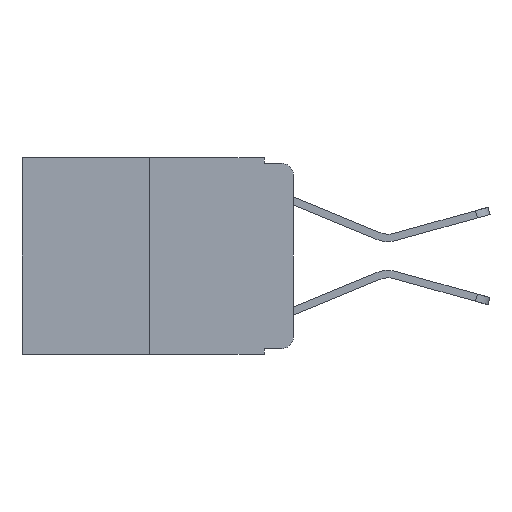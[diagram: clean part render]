
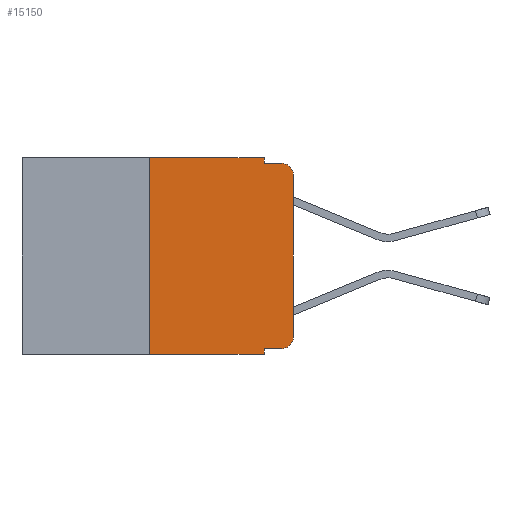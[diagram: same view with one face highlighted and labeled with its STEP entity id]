
A CAD part, left-side view. The second image highlights one B-rep face of the part: STEP entity #15150.
In plain terms, the highlighted planar face has unit normal (-1, 0, 0).
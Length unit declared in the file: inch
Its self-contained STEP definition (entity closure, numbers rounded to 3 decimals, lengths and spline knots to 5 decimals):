
#358 = FACE_OUTER_BOUND ( 'NONE', #2699, .T. ) ;
#746 = CARTESIAN_POINT ( 'NONE',  ( 0., 0., -0.03 ) ) ;
#933 = VECTOR ( 'NONE', #9286, 39.37008 ) ;
#1063 = VERTEX_POINT ( 'NONE', #14488 ) ;
#1134 = CARTESIAN_POINT ( 'NONE',  ( 0., 0.051, -0.01 ) ) ;
#1545 = VERTEX_POINT ( 'NONE', #13090 ) ;
#1669 = ORIENTED_EDGE ( 'NONE', *, *, #3342, .F. ) ;
#2285 = DIRECTION ( 'NONE',  ( 0., -1., 0. ) ) ;
#2361 = CARTESIAN_POINT ( 'NONE',  ( 0., 0.051, -0.343 ) ) ;
#2459 = VERTEX_POINT ( 'NONE', #11951 ) ;
#2699 = EDGE_LOOP ( 'NONE', ( #15648, #10214, #8199, #13859, #8442, #6849, #11143, #1669, #5261, #14802 ) ) ;
#2815 = CARTESIAN_POINT ( 'NONE',  ( 0., 0.25, 0. ) ) ;
#2827 = VECTOR ( 'NONE', #3890, 39.37008 ) ;
#3004 = VECTOR ( 'NONE', #3378, 39.37008 ) ;
#3108 = CARTESIAN_POINT ( 'NONE',  ( 0., 0.473, 0. ) ) ;
#3288 = LINE ( 'NONE', #3391, #2827 ) ;
#3289 = LINE ( 'NONE', #15414, #18353 ) ;
#3342 = EDGE_CURVE ( 'NONE', #17640, #17382, #3288, .T. ) ;
#3378 = DIRECTION ( 'NONE',  ( 0., -1., 0. ) ) ;
#3391 = CARTESIAN_POINT ( 'NONE',  ( 0., 0.051, 0. ) ) ;
#3419 = CARTESIAN_POINT ( 'NONE',  ( 0., 0.051, -0.333 ) ) ;
#3674 = VECTOR ( 'NONE', #11864, 39.37008 ) ;
#3890 = DIRECTION ( 'NONE',  ( 0., 0., -1. ) ) ;
#3921 = VERTEX_POINT ( 'NONE', #12696 ) ;
#4242 = EDGE_CURVE ( 'NONE', #14342, #2459, #15188, .T. ) ;
#4639 = DIRECTION ( 'NONE',  ( 0., 0., -1. ) ) ;
#4884 = AXIS2_PLACEMENT_3D ( 'NONE', #5359, #15498, #6832 ) ;
#4999 = CIRCLE ( 'NONE', #16912, 0.02 ) ;
#5261 = ORIENTED_EDGE ( 'NONE', *, *, #16424, .T. ) ;
#5298 = LINE ( 'NONE', #17523, #16865 ) ;
#5359 = CARTESIAN_POINT ( 'NONE',  ( 0., 0.02, -0.313 ) ) ;
#5643 = EDGE_CURVE ( 'NONE', #11646, #17382, #14668, .T. ) ;
#6179 = VECTOR ( 'NONE', #17844, 39.37008 ) ;
#6579 = CARTESIAN_POINT ( 'NONE',  ( 0., 0.02, -0.03 ) ) ;
#6627 = LINE ( 'NONE', #7706, #6179 ) ;
#6832 = DIRECTION ( 'NONE',  ( 0., 0., -1. ) ) ;
#6849 = ORIENTED_EDGE ( 'NONE', *, *, #7326, .F. ) ;
#7065 = CIRCLE ( 'NONE', #4884, 0.02 ) ;
#7326 = EDGE_CURVE ( 'NONE', #11646, #14342, #5298, .T. ) ;
#7594 = CARTESIAN_POINT ( 'NONE',  ( 0., 0.473, 0. ) ) ;
#7706 = CARTESIAN_POINT ( 'NONE',  ( 0., 0., 0. ) ) ;
#8043 = DIRECTION ( 'NONE',  ( 0., 0., -1. ) ) ;
#8199 = ORIENTED_EDGE ( 'NONE', *, *, #14121, .F. ) ;
#8440 = LINE ( 'NONE', #3419, #933 ) ;
#8442 = ORIENTED_EDGE ( 'NONE', *, *, #4242, .F. ) ;
#8975 = CARTESIAN_POINT ( 'NONE',  ( 0., 0.473, -0.343 ) ) ;
#9242 = EDGE_CURVE ( 'NONE', #3921, #15305, #6627, .T. ) ;
#9286 = DIRECTION ( 'NONE',  ( 0., -1., 0. ) ) ;
#9549 = CARTESIAN_POINT ( 'NONE',  ( 0., 0.25, -0.343 ) ) ;
#10214 = ORIENTED_EDGE ( 'NONE', *, *, #13421, .T. ) ;
#10243 = EDGE_CURVE ( 'NONE', #2459, #17505, #11917, .T. ) ;
#10300 = DIRECTION ( 'NONE',  ( 0., 0., 1. ) ) ;
#11143 = ORIENTED_EDGE ( 'NONE', *, *, #5643, .T. ) ;
#11335 = VECTOR ( 'NONE', #16847, 39.37008 ) ;
#11646 = VERTEX_POINT ( 'NONE', #9549 ) ;
#11864 = DIRECTION ( 'NONE',  ( 0., 0., -1. ) ) ;
#11894 = PLANE ( 'NONE',  #12833 ) ;
#11917 = LINE ( 'NONE', #14787, #3674 ) ;
#11951 = CARTESIAN_POINT ( 'NONE',  ( 0., 0.051, 0. ) ) ;
#12696 = CARTESIAN_POINT ( 'NONE',  ( 0., 0., -0.313 ) ) ;
#12833 = AXIS2_PLACEMENT_3D ( 'NONE', #3108, #13369, #4639 ) ;
#13090 = CARTESIAN_POINT ( 'NONE',  ( 0., 0.02, -0.333 ) ) ;
#13369 = DIRECTION ( 'NONE',  ( 1., 0., 0. ) ) ;
#13421 = EDGE_CURVE ( 'NONE', #15305, #1063, #4999, .T. ) ;
#13523 = EDGE_CURVE ( 'NONE', #1545, #3921, #7065, .T. ) ;
#13859 = ORIENTED_EDGE ( 'NONE', *, *, #10243, .F. ) ;
#14121 = EDGE_CURVE ( 'NONE', #17505, #1063, #3289, .T. ) ;
#14342 = VERTEX_POINT ( 'NONE', #2815 ) ;
#14488 = CARTESIAN_POINT ( 'NONE',  ( 0., 0.02, -0.01 ) ) ;
#14668 = LINE ( 'NONE', #8975, #3004 ) ;
#14705 = CARTESIAN_POINT ( 'NONE',  ( 0., 0.051, -0.333 ) ) ;
#14787 = CARTESIAN_POINT ( 'NONE',  ( 0., 0.051, 0. ) ) ;
#14802 = ORIENTED_EDGE ( 'NONE', *, *, #13523, .T. ) ;
#15150 = ADVANCED_FACE ( 'NONE', ( #358 ), #11894, .F. ) ;
#15188 = LINE ( 'NONE', #7594, #11335 ) ;
#15305 = VERTEX_POINT ( 'NONE', #746 ) ;
#15414 = CARTESIAN_POINT ( 'NONE',  ( 0., 0.051, -0.01 ) ) ;
#15498 = DIRECTION ( 'NONE',  ( -1., 0., 0. ) ) ;
#15648 = ORIENTED_EDGE ( 'NONE', *, *, #9242, .T. ) ;
#16424 = EDGE_CURVE ( 'NONE', #17640, #1545, #8440, .T. ) ;
#16708 = DIRECTION ( 'NONE',  ( -1., 0., 0. ) ) ;
#16847 = DIRECTION ( 'NONE',  ( 0., -1., 0. ) ) ;
#16865 = VECTOR ( 'NONE', #10300, 39.37008 ) ;
#16912 = AXIS2_PLACEMENT_3D ( 'NONE', #6579, #16708, #8043 ) ;
#17382 = VERTEX_POINT ( 'NONE', #2361 ) ;
#17505 = VERTEX_POINT ( 'NONE', #1134 ) ;
#17523 = CARTESIAN_POINT ( 'NONE',  ( 0., 0.25, 0. ) ) ;
#17640 = VERTEX_POINT ( 'NONE', #14705 ) ;
#17844 = DIRECTION ( 'NONE',  ( 0., 0., 1. ) ) ;
#18353 = VECTOR ( 'NONE', #2285, 39.37008 ) ;
